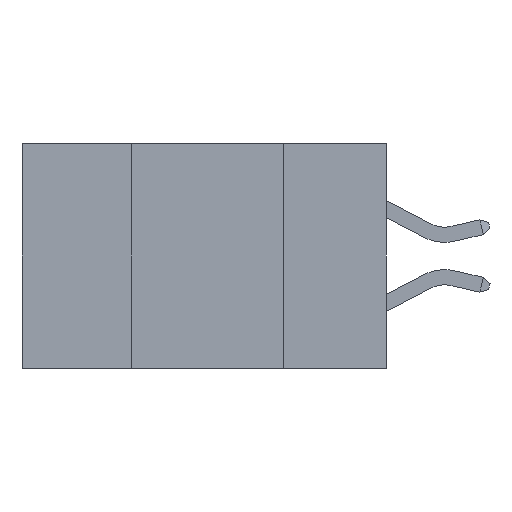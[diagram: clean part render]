
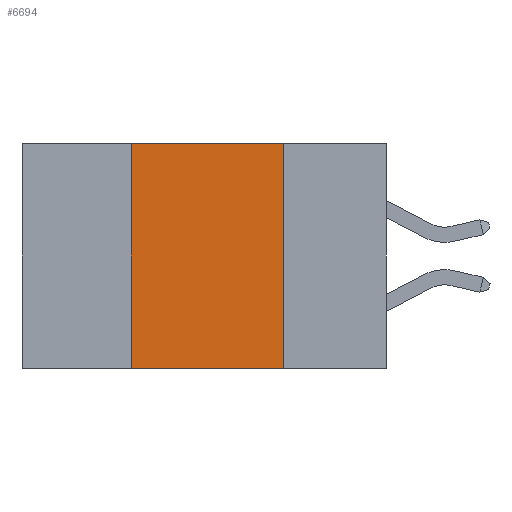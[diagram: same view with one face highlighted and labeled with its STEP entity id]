
A CAD part, left-side view. The second image highlights one B-rep face of the part: STEP entity #6694.
In plain terms, the highlighted planar face has unit normal (-1, 0, 0).
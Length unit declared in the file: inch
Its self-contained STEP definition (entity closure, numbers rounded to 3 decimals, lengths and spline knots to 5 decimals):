
#531 = ORIENTED_EDGE ( 'NONE', *, *, #870, .F. ) ;
#870 = EDGE_CURVE ( 'NONE', #5829, #2437, #8639, .T. ) ;
#2005 = CARTESIAN_POINT ( 'NONE',  ( 0., 0.6, 0. ) ) ;
#2437 = VERTEX_POINT ( 'NONE', #12450 ) ;
#3608 = PLANE ( 'NONE',  #5410 ) ;
#3848 = CARTESIAN_POINT ( 'NONE',  ( 0., 0.42, -0.37 ) ) ;
#4307 = CARTESIAN_POINT ( 'NONE',  ( 0., 0.6, 0. ) ) ;
#4395 = DIRECTION ( 'NONE',  ( 1., 0., 0. ) ) ;
#4429 = VERTEX_POINT ( 'NONE', #3848 ) ;
#4452 = DIRECTION ( 'NONE',  ( 0., 0., -1. ) ) ;
#4632 = EDGE_CURVE ( 'NONE', #2437, #19029, #18200, .T. ) ;
#5410 = AXIS2_PLACEMENT_3D ( 'NONE', #4307, #4395, #4452 ) ;
#5798 = LINE ( 'NONE', #18454, #20007 ) ;
#5829 = VERTEX_POINT ( 'NONE', #9750 ) ;
#6010 = DIRECTION ( 'NONE',  ( 0., 0., 1. ) ) ;
#6694 = ADVANCED_FACE ( 'NONE', ( #12586 ), #3608, .F. ) ;
#6971 = CARTESIAN_POINT ( 'NONE',  ( 0., 0.17, -0.37 ) ) ;
#8639 = LINE ( 'NONE', #2005, #18670 ) ;
#9077 = CARTESIAN_POINT ( 'NONE',  ( 0., 0.17, -0.37 ) ) ;
#9750 = CARTESIAN_POINT ( 'NONE',  ( 0., 0.42, 0. ) ) ;
#10090 = DIRECTION ( 'NONE',  ( 0., -1., 0. ) ) ;
#10143 = LINE ( 'NONE', #10325, #19055 ) ;
#10325 = CARTESIAN_POINT ( 'NONE',  ( 0., 0.6, -0.37 ) ) ;
#11058 = EDGE_CURVE ( 'NONE', #4429, #19029, #10143, .T. ) ;
#11222 = EDGE_LOOP ( 'NONE', ( #21858, #531, #20201, #13287 ) ) ;
#12450 = CARTESIAN_POINT ( 'NONE',  ( 0., 0.17, 0. ) ) ;
#12586 = FACE_OUTER_BOUND ( 'NONE', #11222, .T. ) ;
#12645 = DIRECTION ( 'NONE',  ( 0., -1., 0. ) ) ;
#13287 = ORIENTED_EDGE ( 'NONE', *, *, #11058, .T. ) ;
#14637 = DIRECTION ( 'NONE',  ( 0., 0., -1. ) ) ;
#18200 = LINE ( 'NONE', #9077, #18763 ) ;
#18454 = CARTESIAN_POINT ( 'NONE',  ( 0., 0.42, -0.37 ) ) ;
#18670 = VECTOR ( 'NONE', #12645, 39.37008 ) ;
#18763 = VECTOR ( 'NONE', #14637, 39.37008 ) ;
#19029 = VERTEX_POINT ( 'NONE', #6971 ) ;
#19055 = VECTOR ( 'NONE', #10090, 39.37008 ) ;
#19395 = EDGE_CURVE ( 'NONE', #4429, #5829, #5798, .T. ) ;
#20007 = VECTOR ( 'NONE', #6010, 39.37008 ) ;
#20201 = ORIENTED_EDGE ( 'NONE', *, *, #19395, .F. ) ;
#21858 = ORIENTED_EDGE ( 'NONE', *, *, #4632, .F. ) ;
